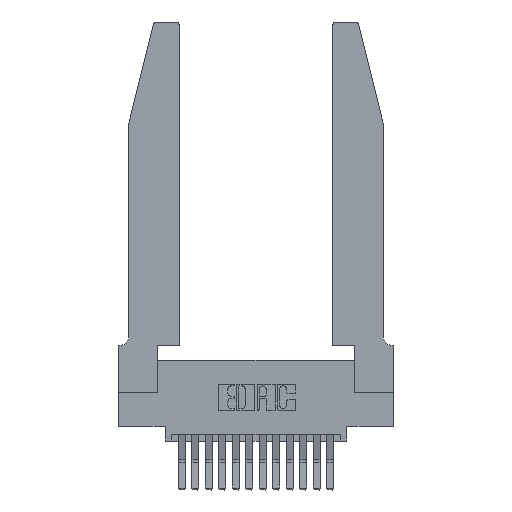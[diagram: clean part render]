
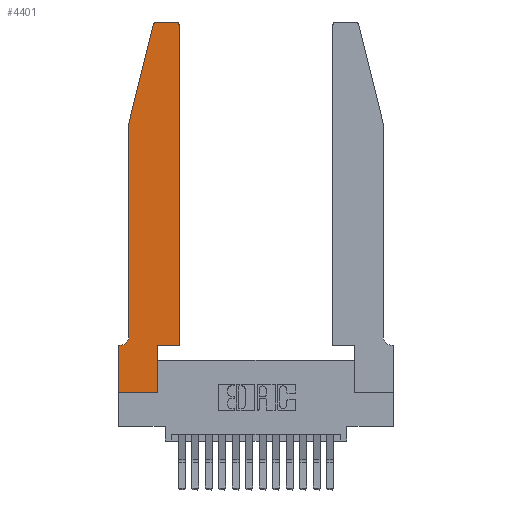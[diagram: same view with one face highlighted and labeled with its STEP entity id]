
A CAD part, top view. The second image highlights one B-rep face of the part: STEP entity #4401.
In plain terms, the highlighted planar face has unit normal (0, 0, 1).
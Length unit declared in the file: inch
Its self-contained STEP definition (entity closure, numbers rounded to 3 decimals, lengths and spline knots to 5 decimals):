
#244 = VERTEX_POINT ( 'NONE', #9058 ) ;
#432 = DIRECTION ( 'NONE',  ( 0., -1., 0. ) ) ;
#465 = DIRECTION ( 'NONE',  ( 1., 0., 0. ) ) ;
#483 = EDGE_CURVE ( 'NONE', #655, #244, #8746, .T. ) ;
#655 = VERTEX_POINT ( 'NONE', #6872 ) ;
#766 = EDGE_LOOP ( 'NONE', ( #12321, #2044, #13582, #14687, #8870, #18393, #4794, #6173, #8630, #5029, #8571, #3890 ) ) ;
#906 = CARTESIAN_POINT ( 'NONE',  ( 0., 0., 0.37 ) ) ;
#994 = CIRCLE ( 'NONE', #12640, 0.07 ) ;
#1009 = CARTESIAN_POINT ( 'NONE',  ( 0.0055, 0.42, 0.37 ) ) ;
#1206 = DIRECTION ( 'NONE',  ( 1., 0., 0. ) ) ;
#2044 = ORIENTED_EDGE ( 'NONE', *, *, #6298, .T. ) ;
#2090 = AXIS2_PLACEMENT_3D ( 'NONE', #5492, #15258, #6957 ) ;
#2343 = VERTEX_POINT ( 'NONE', #12190 ) ;
#2459 = FACE_OUTER_BOUND ( 'NONE', #766, .T. ) ;
#2473 = CARTESIAN_POINT ( 'NONE',  ( 0.284, 2.75, 0.37 ) ) ;
#2508 = DIRECTION ( 'NONE',  ( -1., 0., 0. ) ) ;
#2915 = LINE ( 'NONE', #9779, #10080 ) ;
#3854 = CARTESIAN_POINT ( 'NONE',  ( 0.2865, 0., 0.37 ) ) ;
#3872 = DIRECTION ( 'NONE',  ( -0.239, -0.971, 0. ) ) ;
#3890 = ORIENTED_EDGE ( 'NONE', *, *, #6004, .T. ) ;
#4065 = LINE ( 'NONE', #7727, #14842 ) ;
#4126 = CARTESIAN_POINT ( 'NONE',  ( 0., 0.35, 0.37 ) ) ;
#4200 = CARTESIAN_POINT ( 'NONE',  ( 0.2865, 0.35, 0.37 ) ) ;
#4401 = ADVANCED_FACE ( 'NONE', ( #2459 ), #16773, .T. ) ;
#4432 = AXIS2_PLACEMENT_3D ( 'NONE', #17507, #9150, #465 ) ;
#4699 = LINE ( 'NONE', #13661, #15448 ) ;
#4794 = ORIENTED_EDGE ( 'NONE', *, *, #13464, .T. ) ;
#4847 = VECTOR ( 'NONE', #17265, 39.37008 ) ;
#5029 = ORIENTED_EDGE ( 'NONE', *, *, #6188, .T. ) ;
#5492 = CARTESIAN_POINT ( 'NONE',  ( 0.284, 2.72, 0.37 ) ) ;
#5583 = VECTOR ( 'NONE', #18048, 39.37008 ) ;
#6004 = EDGE_CURVE ( 'NONE', #244, #2343, #7436, .T. ) ;
#6010 = EDGE_CURVE ( 'NONE', #2343, #7347, #14384, .T. ) ;
#6173 = ORIENTED_EDGE ( 'NONE', *, *, #10140, .T. ) ;
#6188 = EDGE_CURVE ( 'NONE', #16870, #655, #4699, .T. ) ;
#6298 = EDGE_CURVE ( 'NONE', #7347, #10899, #10477, .T. ) ;
#6512 = CARTESIAN_POINT ( 'NONE',  ( 0.0755, 0.42, 0.37 ) ) ;
#6871 = VERTEX_POINT ( 'NONE', #3854 ) ;
#6872 = CARTESIAN_POINT ( 'NONE',  ( 0.4505, 0.35, 0.37 ) ) ;
#6957 = DIRECTION ( 'NONE',  ( 1., 0., 0. ) ) ;
#7059 = LINE ( 'NONE', #12740, #14446 ) ;
#7347 = VERTEX_POINT ( 'NONE', #2473 ) ;
#7436 = CIRCLE ( 'NONE', #4432, 0.03 ) ;
#7727 = CARTESIAN_POINT ( 'NONE',  ( 0., 0., 0.37 ) ) ;
#7762 = CARTESIAN_POINT ( 'NONE',  ( 0.2605, 2.75, 0.37 ) ) ;
#8224 = CARTESIAN_POINT ( 'NONE',  ( 0.0055, 0.35, 0.37 ) ) ;
#8305 = VERTEX_POINT ( 'NONE', #16073 ) ;
#8571 = ORIENTED_EDGE ( 'NONE', *, *, #483, .T. ) ;
#8630 = ORIENTED_EDGE ( 'NONE', *, *, #15753, .T. ) ;
#8642 = LINE ( 'NONE', #15838, #4847 ) ;
#8746 = LINE ( 'NONE', #18177, #15706 ) ;
#8870 = ORIENTED_EDGE ( 'NONE', *, *, #9080, .T. ) ;
#8881 = VERTEX_POINT ( 'NONE', #6512 ) ;
#9058 = CARTESIAN_POINT ( 'NONE',  ( 0.4505, 2.72, 0.37 ) ) ;
#9080 = EDGE_CURVE ( 'NONE', #8881, #16730, #994, .T. ) ;
#9150 = DIRECTION ( 'NONE',  ( 0., 0., 1. ) ) ;
#9779 = CARTESIAN_POINT ( 'NONE',  ( 0.0755, 0.35, 0.37 ) ) ;
#9855 = DIRECTION ( 'NONE',  ( 0., 0., 1. ) ) ;
#10065 = LINE ( 'NONE', #15130, #13341 ) ;
#10080 = VECTOR ( 'NONE', #11188, 39.37008 ) ;
#10140 = EDGE_CURVE ( 'NONE', #11034, #6871, #17181, .T. ) ;
#10383 = CARTESIAN_POINT ( 'NONE',  ( 0.25487, 2.72718, 0.37 ) ) ;
#10477 = CIRCLE ( 'NONE', #2090, 0.03 ) ;
#10703 = VECTOR ( 'NONE', #16074, 39.37008 ) ;
#10899 = VERTEX_POINT ( 'NONE', #10383 ) ;
#11034 = VERTEX_POINT ( 'NONE', #13521 ) ;
#11084 = DIRECTION ( 'NONE',  ( 0., 0., -1. ) ) ;
#11188 = DIRECTION ( 'NONE',  ( -1., 0., 0. ) ) ;
#12190 = CARTESIAN_POINT ( 'NONE',  ( 0.4205, 2.75, 0.37 ) ) ;
#12321 = ORIENTED_EDGE ( 'NONE', *, *, #6010, .T. ) ;
#12640 = AXIS2_PLACEMENT_3D ( 'NONE', #1009, #11084, #2508 ) ;
#12740 = CARTESIAN_POINT ( 'NONE',  ( 0.0755, 2., 0.37 ) ) ;
#12830 = AXIS2_PLACEMENT_3D ( 'NONE', #4126, #9855, #1206 ) ;
#13042 = EDGE_CURVE ( 'NONE', #13044, #8881, #7059, .T. ) ;
#13044 = VERTEX_POINT ( 'NONE', #15259 ) ;
#13274 = DIRECTION ( 'NONE',  ( 0., 1., 0. ) ) ;
#13341 = VECTOR ( 'NONE', #3872, 39.37008 ) ;
#13464 = EDGE_CURVE ( 'NONE', #8305, #11034, #4065, .T. ) ;
#13521 = CARTESIAN_POINT ( 'NONE',  ( 0., 0., 0.37 ) ) ;
#13582 = ORIENTED_EDGE ( 'NONE', *, *, #14916, .T. ) ;
#13661 = CARTESIAN_POINT ( 'NONE',  ( 0.4505, 0.35, 0.37 ) ) ;
#13752 = EDGE_CURVE ( 'NONE', #16730, #8305, #2915, .T. ) ;
#14110 = DIRECTION ( 'NONE',  ( 0., -1., 0. ) ) ;
#14384 = LINE ( 'NONE', #7762, #10703 ) ;
#14446 = VECTOR ( 'NONE', #14110, 39.37008 ) ;
#14687 = ORIENTED_EDGE ( 'NONE', *, *, #13042, .T. ) ;
#14842 = VECTOR ( 'NONE', #432, 39.37008 ) ;
#14916 = EDGE_CURVE ( 'NONE', #10899, #13044, #10065, .T. ) ;
#15130 = CARTESIAN_POINT ( 'NONE',  ( 0.0755, 2., 0.37 ) ) ;
#15258 = DIRECTION ( 'NONE',  ( 0., 0., 1. ) ) ;
#15259 = CARTESIAN_POINT ( 'NONE',  ( 0.0755, 2., 0.37 ) ) ;
#15448 = VECTOR ( 'NONE', #16369, 39.37008 ) ;
#15706 = VECTOR ( 'NONE', #13274, 39.37008 ) ;
#15753 = EDGE_CURVE ( 'NONE', #6871, #16870, #8642, .T. ) ;
#15838 = CARTESIAN_POINT ( 'NONE',  ( 0.2865, 0.35, 0.37 ) ) ;
#16073 = CARTESIAN_POINT ( 'NONE',  ( 0., 0.35, 0.37 ) ) ;
#16074 = DIRECTION ( 'NONE',  ( -1., 0., 0. ) ) ;
#16369 = DIRECTION ( 'NONE',  ( 1., 0., 0. ) ) ;
#16730 = VERTEX_POINT ( 'NONE', #8224 ) ;
#16773 = PLANE ( 'NONE',  #12830 ) ;
#16870 = VERTEX_POINT ( 'NONE', #4200 ) ;
#17181 = LINE ( 'NONE', #906, #5583 ) ;
#17265 = DIRECTION ( 'NONE',  ( 0., 1., 0. ) ) ;
#17507 = CARTESIAN_POINT ( 'NONE',  ( 0.4205, 2.72, 0.37 ) ) ;
#18048 = DIRECTION ( 'NONE',  ( 1., 0., 0. ) ) ;
#18177 = CARTESIAN_POINT ( 'NONE',  ( 0.4505, 0.35, 0.37 ) ) ;
#18393 = ORIENTED_EDGE ( 'NONE', *, *, #13752, .T. ) ;
